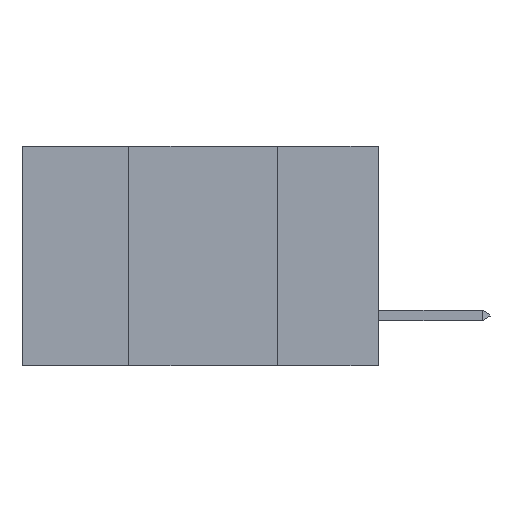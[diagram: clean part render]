
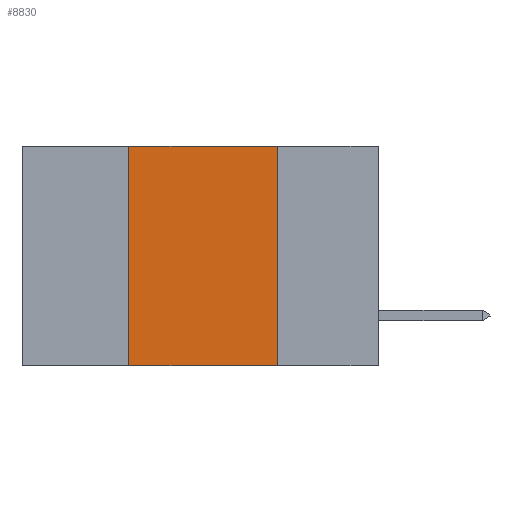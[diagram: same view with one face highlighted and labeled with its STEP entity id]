
A CAD part, left-side view. The second image highlights one B-rep face of the part: STEP entity #8830.
In plain terms, the highlighted planar face has unit normal (-1, 0, 0).
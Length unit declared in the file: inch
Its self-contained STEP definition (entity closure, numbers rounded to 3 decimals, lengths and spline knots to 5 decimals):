
#19 = DIRECTION ( 'NONE',  ( 0., 0., -1. ) ) ;
#30 = CARTESIAN_POINT ( 'NONE',  ( 0., 0.42, -0.37 ) ) ;
#234 = EDGE_CURVE ( 'NONE', #7030, #13993, #3650, .T. ) ;
#269 = EDGE_CURVE ( 'NONE', #7030, #781, #4868, .T. ) ;
#344 = LINE ( 'NONE', #6911, #7819 ) ;
#781 = VERTEX_POINT ( 'NONE', #1505 ) ;
#1121 = PLANE ( 'NONE',  #11737 ) ;
#1168 = ORIENTED_EDGE ( 'NONE', *, *, #12779, .F. ) ;
#1169 = CARTESIAN_POINT ( 'NONE',  ( 0., 0.42, 0. ) ) ;
#1505 = CARTESIAN_POINT ( 'NONE',  ( 0., 0.17, -0.37 ) ) ;
#2218 = DIRECTION ( 'NONE',  ( 1., 0., 0. ) ) ;
#2883 = DIRECTION ( 'NONE',  ( 0., -1., 0. ) ) ;
#3650 = LINE ( 'NONE', #1169, #9184 ) ;
#4182 = VECTOR ( 'NONE', #2883, 39.37008 ) ;
#4234 = ORIENTED_EDGE ( 'NONE', *, *, #234, .F. ) ;
#4639 = CARTESIAN_POINT ( 'NONE',  ( 0., 0.6, -0.37 ) ) ;
#4868 = LINE ( 'NONE', #4639, #11415 ) ;
#5217 = CARTESIAN_POINT ( 'NONE',  ( 0., 0.6, 0. ) ) ;
#6230 = EDGE_CURVE ( 'NONE', #10009, #781, #344, .T. ) ;
#6513 = CARTESIAN_POINT ( 'NONE',  ( 0., 0.17, 0. ) ) ;
#6911 = CARTESIAN_POINT ( 'NONE',  ( 0., 0.17, 0. ) ) ;
#7030 = VERTEX_POINT ( 'NONE', #30 ) ;
#7489 = ORIENTED_EDGE ( 'NONE', *, *, #269, .T. ) ;
#7819 = VECTOR ( 'NONE', #8222, 39.37008 ) ;
#8222 = DIRECTION ( 'NONE',  ( 0., 0., -1. ) ) ;
#8830 = ADVANCED_FACE ( 'NONE', ( #12402 ), #1121, .F. ) ;
#8842 = CARTESIAN_POINT ( 'NONE',  ( 0., 0.6, 0. ) ) ;
#9184 = VECTOR ( 'NONE', #12233, 39.37008 ) ;
#9188 = LINE ( 'NONE', #5217, #4182 ) ;
#10009 = VERTEX_POINT ( 'NONE', #6513 ) ;
#11397 = EDGE_LOOP ( 'NONE', ( #11859, #1168, #4234, #7489 ) ) ;
#11415 = VECTOR ( 'NONE', #12207, 39.37008 ) ;
#11737 = AXIS2_PLACEMENT_3D ( 'NONE', #8842, #2218, #19 ) ;
#11859 = ORIENTED_EDGE ( 'NONE', *, *, #6230, .F. ) ;
#12207 = DIRECTION ( 'NONE',  ( 0., -1., 0. ) ) ;
#12233 = DIRECTION ( 'NONE',  ( 0., 0., 1. ) ) ;
#12402 = FACE_OUTER_BOUND ( 'NONE', #11397, .T. ) ;
#12779 = EDGE_CURVE ( 'NONE', #13993, #10009, #9188, .T. ) ;
#13993 = VERTEX_POINT ( 'NONE', #14097 ) ;
#14097 = CARTESIAN_POINT ( 'NONE',  ( 0., 0.42, 0. ) ) ;
